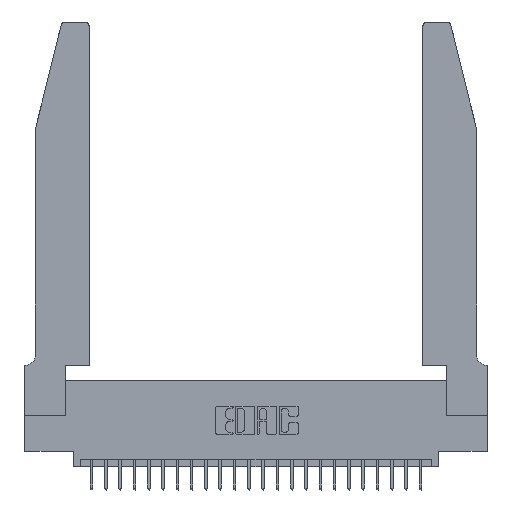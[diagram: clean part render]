
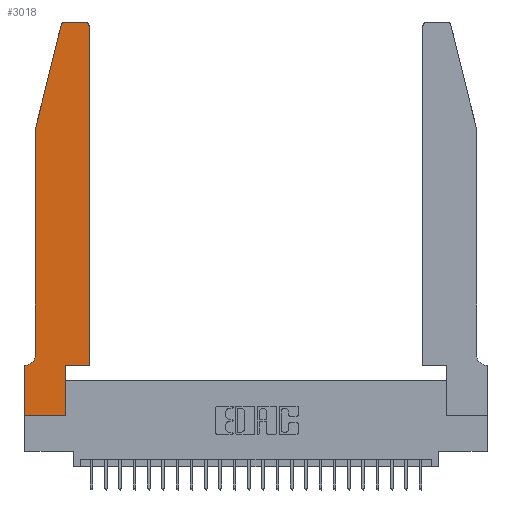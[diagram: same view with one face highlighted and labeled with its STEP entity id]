
A CAD part, top view. The second image highlights one B-rep face of the part: STEP entity #3018.
In plain terms, the highlighted planar face has unit normal (0, 0, 1).
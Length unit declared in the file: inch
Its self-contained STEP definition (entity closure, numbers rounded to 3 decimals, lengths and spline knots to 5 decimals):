
#96 = ORIENTED_EDGE ( 'NONE', *, *, #10783, .T. ) ;
#299 = EDGE_CURVE ( 'NONE', #17544, #2565, #4740, .T. ) ;
#907 = ORIENTED_EDGE ( 'NONE', *, *, #9672, .T. ) ;
#1240 = ORIENTED_EDGE ( 'NONE', *, *, #299, .T. ) ;
#1367 = CARTESIAN_POINT ( 'NONE',  ( 0., 0., 0.37 ) ) ;
#1536 = LINE ( 'NONE', #19348, #22170 ) ;
#2303 = VERTEX_POINT ( 'NONE', #23684 ) ;
#2323 = DIRECTION ( 'NONE',  ( 1., 0., 0. ) ) ;
#2415 = VECTOR ( 'NONE', #14840, 39.37008 ) ;
#2565 = VERTEX_POINT ( 'NONE', #21056 ) ;
#3018 = ADVANCED_FACE ( 'NONE', ( #6671 ), #21855, .T. ) ;
#3091 = LINE ( 'NONE', #13068, #16408 ) ;
#3110 = CARTESIAN_POINT ( 'NONE',  ( 0.0055, 0.42, 0.37 ) ) ;
#3337 = EDGE_CURVE ( 'NONE', #14577, #22209, #8886, .T. ) ;
#3368 = CARTESIAN_POINT ( 'NONE',  ( 0.4205, 2.72, 0.37 ) ) ;
#3475 = ORIENTED_EDGE ( 'NONE', *, *, #12716, .T. ) ;
#3642 = DIRECTION ( 'NONE',  ( -1., 0., 0. ) ) ;
#3699 = AXIS2_PLACEMENT_3D ( 'NONE', #10349, #10440, #2323 ) ;
#4406 = AXIS2_PLACEMENT_3D ( 'NONE', #3110, #9438, #9347 ) ;
#4740 = CIRCLE ( 'NONE', #7307, 0.03 ) ;
#4799 = DIRECTION ( 'NONE',  ( 1., 0., 0. ) ) ;
#5363 = EDGE_CURVE ( 'NONE', #12220, #15853, #7554, .T. ) ;
#5459 = VERTEX_POINT ( 'NONE', #24149 ) ;
#5901 = CARTESIAN_POINT ( 'NONE',  ( 0.0755, 0.35, 0.37 ) ) ;
#6671 = FACE_OUTER_BOUND ( 'NONE', #22229, .T. ) ;
#6860 = VECTOR ( 'NONE', #4799, 39.37008 ) ;
#7003 = CIRCLE ( 'NONE', #4406, 0.07 ) ;
#7307 = AXIS2_PLACEMENT_3D ( 'NONE', #3368, #15422, #17461 ) ;
#7325 = LINE ( 'NONE', #23990, #18372 ) ;
#7554 = LINE ( 'NONE', #15896, #12289 ) ;
#7889 = LINE ( 'NONE', #8739, #2415 ) ;
#8477 = ORIENTED_EDGE ( 'NONE', *, *, #24705, .T. ) ;
#8527 = CARTESIAN_POINT ( 'NONE',  ( 0.284, 2.75, 0.37 ) ) ;
#8640 = CARTESIAN_POINT ( 'NONE',  ( 0.2865, 0.35, 0.37 ) ) ;
#8739 = CARTESIAN_POINT ( 'NONE',  ( 0., 0., 0.37 ) ) ;
#8886 = CIRCLE ( 'NONE', #3699, 0.03 ) ;
#9347 = DIRECTION ( 'NONE',  ( -1., 0., 0. ) ) ;
#9438 = DIRECTION ( 'NONE',  ( 0., 0., -1. ) ) ;
#9672 = EDGE_CURVE ( 'NONE', #22209, #2303, #14756, .T. ) ;
#9728 = DIRECTION ( 'NONE',  ( 0., 0., 1. ) ) ;
#9832 = DIRECTION ( 'NONE',  ( 1., 0., 0. ) ) ;
#10349 = CARTESIAN_POINT ( 'NONE',  ( 0.284, 2.72, 0.37 ) ) ;
#10440 = DIRECTION ( 'NONE',  ( 0., 0., 1. ) ) ;
#10677 = ORIENTED_EDGE ( 'NONE', *, *, #20859, .T. ) ;
#10732 = CARTESIAN_POINT ( 'NONE',  ( 0.2605, 2.75, 0.37 ) ) ;
#10783 = EDGE_CURVE ( 'NONE', #2565, #14577, #21690, .T. ) ;
#11162 = CARTESIAN_POINT ( 'NONE',  ( 0.0055, 0.35, 0.37 ) ) ;
#11882 = DIRECTION ( 'NONE',  ( 0., -1., 0. ) ) ;
#12018 = CARTESIAN_POINT ( 'NONE',  ( 0., 0.35, 0.37 ) ) ;
#12220 = VERTEX_POINT ( 'NONE', #1367 ) ;
#12289 = VECTOR ( 'NONE', #9832, 39.37008 ) ;
#12465 = ORIENTED_EDGE ( 'NONE', *, *, #19135, .T. ) ;
#12716 = EDGE_CURVE ( 'NONE', #2303, #5459, #7325, .T. ) ;
#12846 = ORIENTED_EDGE ( 'NONE', *, *, #3337, .T. ) ;
#12940 = CARTESIAN_POINT ( 'NONE',  ( 0.2865, 0., 0.37 ) ) ;
#13010 = ORIENTED_EDGE ( 'NONE', *, *, #13336, .T. ) ;
#13068 = CARTESIAN_POINT ( 'NONE',  ( 0.2865, 0.35, 0.37 ) ) ;
#13291 = VECTOR ( 'NONE', #3642, 39.37008 ) ;
#13336 = EDGE_CURVE ( 'NONE', #20999, #17544, #1536, .T. ) ;
#13790 = DIRECTION ( 'NONE',  ( -1., 0., 0. ) ) ;
#14466 = VERTEX_POINT ( 'NONE', #11162 ) ;
#14577 = VERTEX_POINT ( 'NONE', #8527 ) ;
#14756 = LINE ( 'NONE', #20753, #26161 ) ;
#14838 = ORIENTED_EDGE ( 'NONE', *, *, #5363, .T. ) ;
#14840 = DIRECTION ( 'NONE',  ( 0., -1., 0. ) ) ;
#15422 = DIRECTION ( 'NONE',  ( 0., 0., 1. ) ) ;
#15853 = VERTEX_POINT ( 'NONE', #12940 ) ;
#15896 = CARTESIAN_POINT ( 'NONE',  ( 0., 0., 0.37 ) ) ;
#15980 = CARTESIAN_POINT ( 'NONE',  ( 0.4505, 2.72, 0.37 ) ) ;
#16408 = VECTOR ( 'NONE', #16932, 39.37008 ) ;
#16524 = CARTESIAN_POINT ( 'NONE',  ( 0.25487, 2.72718, 0.37 ) ) ;
#16932 = DIRECTION ( 'NONE',  ( 0., 1., 0. ) ) ;
#16966 = ORIENTED_EDGE ( 'NONE', *, *, #25853, .T. ) ;
#17461 = DIRECTION ( 'NONE',  ( 1., 0., 0. ) ) ;
#17544 = VERTEX_POINT ( 'NONE', #15980 ) ;
#17839 = VERTEX_POINT ( 'NONE', #20101 ) ;
#18372 = VECTOR ( 'NONE', #11882, 39.37008 ) ;
#18713 = CARTESIAN_POINT ( 'NONE',  ( 0.4505, 0.35, 0.37 ) ) ;
#19135 = EDGE_CURVE ( 'NONE', #17839, #12220, #7889, .T. ) ;
#19299 = LINE ( 'NONE', #5901, #13291 ) ;
#19348 = CARTESIAN_POINT ( 'NONE',  ( 0.4505, 0.35, 0.37 ) ) ;
#19688 = DIRECTION ( 'NONE',  ( -0.239, -0.971, 0. ) ) ;
#20101 = CARTESIAN_POINT ( 'NONE',  ( 0., 0.35, 0.37 ) ) ;
#20395 = VECTOR ( 'NONE', #13790, 39.37008 ) ;
#20753 = CARTESIAN_POINT ( 'NONE',  ( 0.0755, 2., 0.37 ) ) ;
#20859 = EDGE_CURVE ( 'NONE', #20959, #20999, #25187, .T. ) ;
#20959 = VERTEX_POINT ( 'NONE', #8640 ) ;
#20999 = VERTEX_POINT ( 'NONE', #21038 ) ;
#21038 = CARTESIAN_POINT ( 'NONE',  ( 0.4505, 0.35, 0.37 ) ) ;
#21056 = CARTESIAN_POINT ( 'NONE',  ( 0.4205, 2.75, 0.37 ) ) ;
#21690 = LINE ( 'NONE', #10732, #20395 ) ;
#21771 = DIRECTION ( 'NONE',  ( 1., 0., 0. ) ) ;
#21855 = PLANE ( 'NONE',  #22252 ) ;
#22170 = VECTOR ( 'NONE', #24780, 39.37008 ) ;
#22209 = VERTEX_POINT ( 'NONE', #16524 ) ;
#22229 = EDGE_LOOP ( 'NONE', ( #96, #12846, #907, #3475, #8477, #23644, #12465, #14838, #16966, #10677, #13010, #1240 ) ) ;
#22252 = AXIS2_PLACEMENT_3D ( 'NONE', #12018, #9728, #21771 ) ;
#23644 = ORIENTED_EDGE ( 'NONE', *, *, #25294, .T. ) ;
#23684 = CARTESIAN_POINT ( 'NONE',  ( 0.0755, 2., 0.37 ) ) ;
#23990 = CARTESIAN_POINT ( 'NONE',  ( 0.0755, 2., 0.37 ) ) ;
#24149 = CARTESIAN_POINT ( 'NONE',  ( 0.0755, 0.42, 0.37 ) ) ;
#24705 = EDGE_CURVE ( 'NONE', #5459, #14466, #7003, .T. ) ;
#24780 = DIRECTION ( 'NONE',  ( 0., 1., 0. ) ) ;
#25187 = LINE ( 'NONE', #18713, #6860 ) ;
#25294 = EDGE_CURVE ( 'NONE', #14466, #17839, #19299, .T. ) ;
#25853 = EDGE_CURVE ( 'NONE', #15853, #20959, #3091, .T. ) ;
#26161 = VECTOR ( 'NONE', #19688, 39.37008 ) ;
